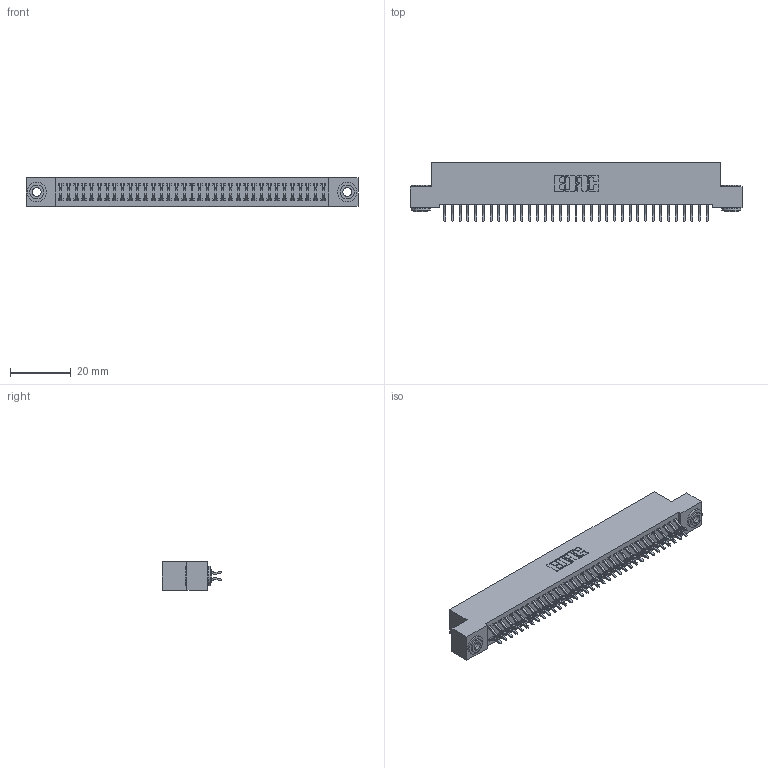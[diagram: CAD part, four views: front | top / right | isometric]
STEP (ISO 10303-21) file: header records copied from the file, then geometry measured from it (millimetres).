
FILE_DESCRIPTION (( 'STEP AP203' ), '1' );
FILE_NAME ('392-070-556-203.STEP', '2018-08-17T23:40:07', ( '' ), ( '' ), 'SwSTEP 2.0', 'SolidWorks 2016', '' );
FILE_SCHEMA (( 'CONFIG_CONTROL_DESIGN' ));
Length unit declared in the file: inch
Products named in the file (4): 345-292-001_556 Tail; 342-250-002_345-250-002-102; 392-070-556-203; 342 Part_.156 TH
Assembly tree (73 placements, depth 2):
  392-070-556-203
    342 Part_.156 TH
    345-292-001_556 Tail  x70
    342-250-002_345-250-002-102  x2
Bounding box: 109.22 x 19.58 x 9.4 mm (x, y, z)
Volume: 9801.3 mm3; surface area: 15927.8 mm2
Topology: 73 solids, 73 shells, 4208 faces, 12485 edges, 8226 vertices
Faces by surface type: plane 2876, cylinder 1324, cone 8
Entity records: 24160 total; most frequent: CARTESIAN_POINT 4001, ORIENTED_EDGE 3918, DIRECTION 3453, EDGE_CURVE 1959, VECTOR 1799, LINE 1799, VERTEX_POINT 1302, AXIS2_PLACEMENT_3D 827
